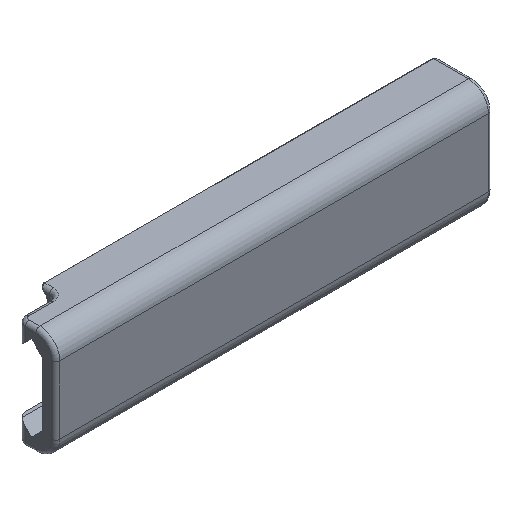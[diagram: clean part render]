
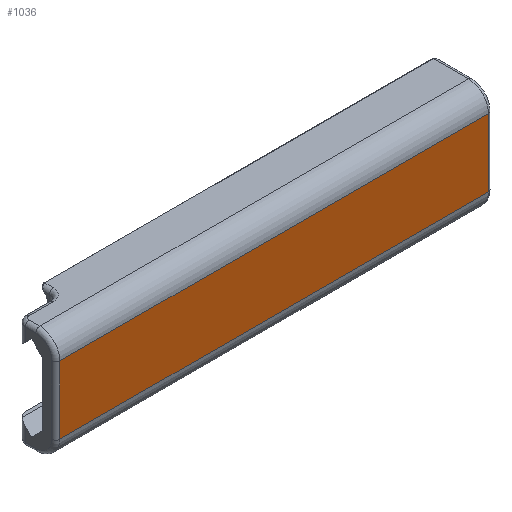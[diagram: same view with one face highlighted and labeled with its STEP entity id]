
A CAD part, isometric view. The second image highlights one B-rep face of the part: STEP entity #1036.
In plain terms, the highlighted planar face has unit normal (0, -1, 0).
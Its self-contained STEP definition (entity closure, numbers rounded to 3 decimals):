
#48=PLANE('',#1170);
#102=FACE_OUTER_BOUND('',#166,.T.);
#166=EDGE_LOOP('',(#855,#856,#857,#858));
#242=LINE('',#2052,#322);
#250=LINE('',#2097,#330);
#251=LINE('',#2101,#331);
#252=LINE('',#2102,#332);
#322=VECTOR('',#1408,10.);
#330=VECTOR('',#1450,10.);
#331=VECTOR('',#1455,10.);
#332=VECTOR('',#1456,10.);
#483=VERTEX_POINT('',#2044);
#485=VERTEX_POINT('',#2050);
#496=VERTEX_POINT('',#2096);
#497=VERTEX_POINT('',#2100);
#610=EDGE_CURVE('',#485,#483,#242,.T.);
#629=EDGE_CURVE('',#483,#496,#250,.T.);
#631=EDGE_CURVE('',#497,#485,#251,.T.);
#632=EDGE_CURVE('',#496,#497,#252,.T.);
#855=ORIENTED_EDGE('',*,*,#610,.F.);
#856=ORIENTED_EDGE('',*,*,#631,.F.);
#857=ORIENTED_EDGE('',*,*,#632,.F.);
#858=ORIENTED_EDGE('',*,*,#629,.F.);
#1036=ADVANCED_FACE('',(#102),#48,.T.);
#1170=AXIS2_PLACEMENT_3D('',#2099,#1453,#1454);
#1408=DIRECTION('',(0.,0.,1.));
#1450=DIRECTION('',(1.,0.,0.));
#1453=DIRECTION('center_axis',(0.,-1.,
0.));
#1454=DIRECTION('ref_axis',(0.,0.,1.));
#1455=DIRECTION('',(-1.,0.,0.));
#1456=DIRECTION('',(0.,0.,-1.));
#2044=CARTESIAN_POINT('',(115.95,-36.854,8.367));
#2050=CARTESIAN_POINT('',(115.95,-36.854,-8.565));
#2052=CARTESIAN_POINT('',(115.95,-36.854,-6.832));
#2096=CARTESIAN_POINT('',(222.918,-36.854,8.367));
#2097=CARTESIAN_POINT('',(223.918,-36.854,8.367));
#2099=CARTESIAN_POINT('Origin',(223.918,-36.854,-13.565));
#2100=CARTESIAN_POINT('',(222.918,-36.854,-8.565));
#2101=CARTESIAN_POINT('',(223.918,-36.854,-8.565));
#2102=CARTESIAN_POINT('',(222.918,-36.854,-6.832));
